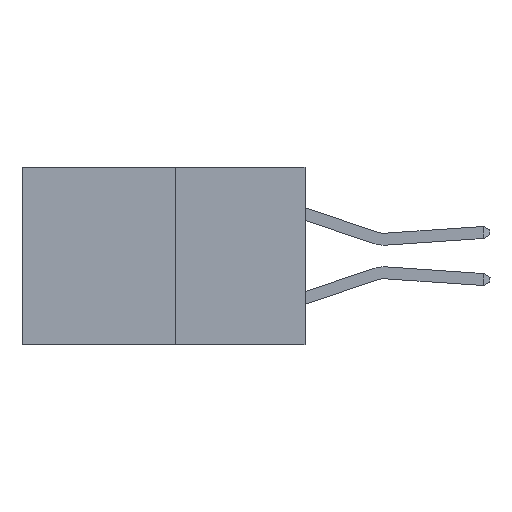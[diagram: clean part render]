
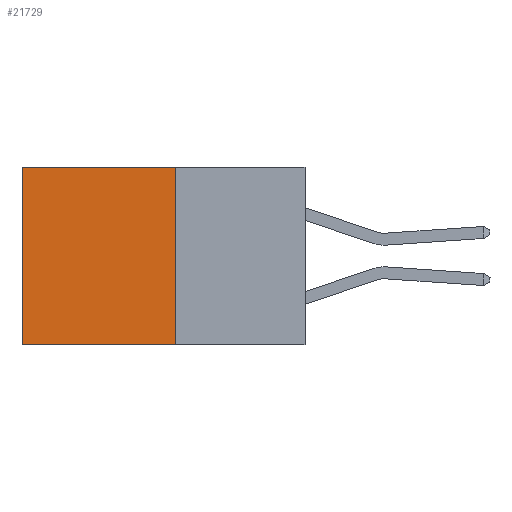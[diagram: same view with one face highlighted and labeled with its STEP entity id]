
A CAD part, left-side view. The second image highlights one B-rep face of the part: STEP entity #21729.
In plain terms, the highlighted planar face has unit normal (-1, 0, 0).
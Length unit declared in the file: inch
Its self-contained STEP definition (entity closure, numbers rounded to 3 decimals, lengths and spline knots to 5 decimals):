
#624 = ORIENTED_EDGE ( 'NONE', *, *, #3488, .F. ) ;
#657 = ORIENTED_EDGE ( 'NONE', *, *, #17735, .T. ) ;
#1208 = VECTOR ( 'NONE', #6813, 39.37008 ) ;
#2012 = VECTOR ( 'NONE', #22257, 39.37008 ) ;
#2305 = ORIENTED_EDGE ( 'NONE', *, *, #19242, .F. ) ;
#2913 = CARTESIAN_POINT ( 'NONE',  ( 0.277, 0.27, -0.37 ) ) ;
#3488 = EDGE_CURVE ( 'NONE', #4690, #18145, #21454, .T. ) ;
#3594 = VERTEX_POINT ( 'NONE', #7833 ) ;
#4164 = CARTESIAN_POINT ( 'NONE',  ( 0.277, 0.27, -0.37 ) ) ;
#4690 = VERTEX_POINT ( 'NONE', #16359 ) ;
#6243 = EDGE_LOOP ( 'NONE', ( #20801, #2305, #624, #657 ) ) ;
#6813 = DIRECTION ( 'NONE',  ( 0., 0., -1. ) ) ;
#7579 = LINE ( 'NONE', #20257, #2012 ) ;
#7833 = CARTESIAN_POINT ( 'NONE',  ( 0.277, 0.59, -0.37 ) ) ;
#8673 = VECTOR ( 'NONE', #23854, 39.37008 ) ;
#9201 = CARTESIAN_POINT ( 'NONE',  ( 0.277, 0.27, -0.37 ) ) ;
#9766 = CARTESIAN_POINT ( 'NONE',  ( 0.277, 0.27, -0.37 ) ) ;
#10328 = VERTEX_POINT ( 'NONE', #12612 ) ;
#11248 = DIRECTION ( 'NONE',  ( 0., 0., -1. ) ) ;
#12612 = CARTESIAN_POINT ( 'NONE',  ( 0.277, 0.59, 0. ) ) ;
#13194 = PLANE ( 'NONE',  #17028 ) ;
#14323 = DIRECTION ( 'NONE',  ( 0., 1., 0. ) ) ;
#16000 = CARTESIAN_POINT ( 'NONE',  ( 0.277, 0.27, 0. ) ) ;
#16359 = CARTESIAN_POINT ( 'NONE',  ( 0.277, 0.27, 0. ) ) ;
#17028 = AXIS2_PLACEMENT_3D ( 'NONE', #9201, #23090, #11248 ) ;
#17735 = EDGE_CURVE ( 'NONE', #4690, #10328, #19253, .T. ) ;
#18145 = VERTEX_POINT ( 'NONE', #2913 ) ;
#19242 = EDGE_CURVE ( 'NONE', #18145, #3594, #19478, .T. ) ;
#19253 = LINE ( 'NONE', #16000, #8673 ) ;
#19478 = LINE ( 'NONE', #4164, #24721 ) ;
#20257 = CARTESIAN_POINT ( 'NONE',  ( 0.277, 0.59, -0.37 ) ) ;
#20801 = ORIENTED_EDGE ( 'NONE', *, *, #24136, .T. ) ;
#21454 = LINE ( 'NONE', #9766, #1208 ) ;
#21729 = ADVANCED_FACE ( 'NONE', ( #24024 ), #13194, .F. ) ;
#22257 = DIRECTION ( 'NONE',  ( 0., 0., -1. ) ) ;
#23090 = DIRECTION ( 'NONE',  ( 1., 0., 0. ) ) ;
#23854 = DIRECTION ( 'NONE',  ( 0., 1., 0. ) ) ;
#24024 = FACE_OUTER_BOUND ( 'NONE', #6243, .T. ) ;
#24136 = EDGE_CURVE ( 'NONE', #10328, #3594, #7579, .T. ) ;
#24721 = VECTOR ( 'NONE', #14323, 39.37008 ) ;
